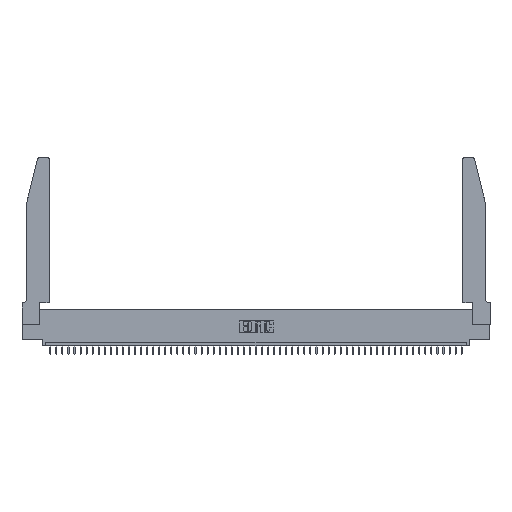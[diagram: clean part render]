
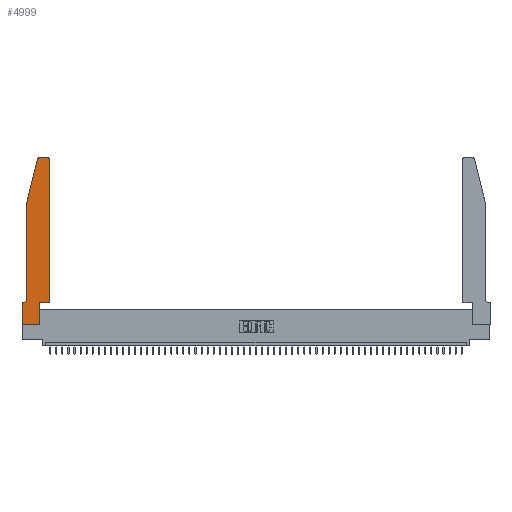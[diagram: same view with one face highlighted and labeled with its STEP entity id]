
A CAD part, top view. The second image highlights one B-rep face of the part: STEP entity #4999.
In plain terms, the highlighted planar face has unit normal (0, 0, 1).
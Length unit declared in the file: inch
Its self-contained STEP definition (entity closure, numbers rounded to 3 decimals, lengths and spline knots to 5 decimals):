
#394 = CARTESIAN_POINT ( 'NONE',  ( 0.0755, 2., 0.37 ) ) ;
#977 = EDGE_CURVE ( 'NONE', #12827, #989, #22823, .T. ) ;
#989 = VERTEX_POINT ( 'NONE', #33174 ) ;
#1142 = AXIS2_PLACEMENT_3D ( 'NONE', #29345, #42253, #9638 ) ;
#1189 = EDGE_CURVE ( 'NONE', #13287, #12827, #1862, .T. ) ;
#1862 = LINE ( 'NONE', #22074, #22867 ) ;
#1951 = DIRECTION ( 'NONE',  ( -1., 0., 0. ) ) ;
#2923 = DIRECTION ( 'NONE',  ( 1., 0., 0. ) ) ;
#4342 = DIRECTION ( 'NONE',  ( 1., 0., 0. ) ) ;
#4626 = VERTEX_POINT ( 'NONE', #16814 ) ;
#4999 = ADVANCED_FACE ( 'NONE', ( #16238 ), #24892, .T. ) ;
#5013 = LINE ( 'NONE', #41927, #43911 ) ;
#5297 = DIRECTION ( 'NONE',  ( -0.239, -0.971, 0. ) ) ;
#5701 = VERTEX_POINT ( 'NONE', #25936 ) ;
#7807 = EDGE_CURVE ( 'NONE', #13977, #37453, #43883, .T. ) ;
#7870 = CARTESIAN_POINT ( 'NONE',  ( 0.4505, 0.35, 0.37 ) ) ;
#8612 = ORIENTED_EDGE ( 'NONE', *, *, #1189, .T. ) ;
#8621 = VERTEX_POINT ( 'NONE', #28650 ) ;
#8873 = EDGE_CURVE ( 'NONE', #20160, #5701, #52295, .T. ) ;
#8943 = ORIENTED_EDGE ( 'NONE', *, *, #35879, .T. ) ;
#9638 = DIRECTION ( 'NONE',  ( 1., 0., 0. ) ) ;
#10596 = EDGE_CURVE ( 'NONE', #41810, #4626, #53225, .T. ) ;
#10607 = CIRCLE ( 'NONE', #1142, 0.03 ) ;
#10634 = VECTOR ( 'NONE', #29252, 39.37008 ) ;
#11757 = CARTESIAN_POINT ( 'NONE',  ( 0., 0., 0.37 ) ) ;
#12827 = VERTEX_POINT ( 'NONE', #26714 ) ;
#13287 = VERTEX_POINT ( 'NONE', #30413 ) ;
#13802 = CARTESIAN_POINT ( 'NONE',  ( 0.4505, 0.35, 0.37 ) ) ;
#13977 = VERTEX_POINT ( 'NONE', #50660 ) ;
#14896 = EDGE_CURVE ( 'NONE', #30742, #8621, #15386, .T. ) ;
#15386 = LINE ( 'NONE', #7870, #46083 ) ;
#16238 = FACE_OUTER_BOUND ( 'NONE', #37562, .T. ) ;
#16446 = CARTESIAN_POINT ( 'NONE',  ( 0., 0., 0.37 ) ) ;
#16768 = AXIS2_PLACEMENT_3D ( 'NONE', #46085, #28875, #4342 ) ;
#16814 = CARTESIAN_POINT ( 'NONE',  ( 0., 0.35, 0.37 ) ) ;
#17313 = LINE ( 'NONE', #13802, #19300 ) ;
#18784 = CARTESIAN_POINT ( 'NONE',  ( 0.0055, 0.35, 0.37 ) ) ;
#19300 = VECTOR ( 'NONE', #49950, 39.37008 ) ;
#20160 = VERTEX_POINT ( 'NONE', #394 ) ;
#20264 = DIRECTION ( 'NONE',  ( 0., 1., 0. ) ) ;
#20481 = VECTOR ( 'NONE', #2923, 39.37008 ) ;
#20873 = ORIENTED_EDGE ( 'NONE', *, *, #977, .T. ) ;
#21095 = DIRECTION ( 'NONE',  ( 1., 0., 0. ) ) ;
#21529 = LINE ( 'NONE', #26131, #34933 ) ;
#22074 = CARTESIAN_POINT ( 'NONE',  ( 0.2605, 2.75, 0.37 ) ) ;
#22645 = EDGE_CURVE ( 'NONE', #5701, #41810, #32778, .T. ) ;
#22823 = CIRCLE ( 'NONE', #16768, 0.03 ) ;
#22867 = VECTOR ( 'NONE', #22886, 39.37008 ) ;
#22886 = DIRECTION ( 'NONE',  ( -1., 0., 0. ) ) ;
#24339 = VECTOR ( 'NONE', #44229, 39.37008 ) ;
#24705 = VECTOR ( 'NONE', #36691, 39.37008 ) ;
#24892 = PLANE ( 'NONE',  #42009 ) ;
#25166 = CARTESIAN_POINT ( 'NONE',  ( 0., 0.35, 0.37 ) ) ;
#25936 = CARTESIAN_POINT ( 'NONE',  ( 0.0755, 0.42, 0.37 ) ) ;
#26131 = CARTESIAN_POINT ( 'NONE',  ( 0.2865, 0.35, 0.37 ) ) ;
#26133 = ORIENTED_EDGE ( 'NONE', *, *, #8873, .T. ) ;
#26192 = CARTESIAN_POINT ( 'NONE',  ( 0.4505, 0.35, 0.37 ) ) ;
#26714 = CARTESIAN_POINT ( 'NONE',  ( 0.284, 2.75, 0.37 ) ) ;
#27071 = EDGE_CURVE ( 'NONE', #989, #20160, #5013, .T. ) ;
#28650 = CARTESIAN_POINT ( 'NONE',  ( 0.4505, 2.72, 0.37 ) ) ;
#28875 = DIRECTION ( 'NONE',  ( 0., 0., 1. ) ) ;
#29252 = DIRECTION ( 'NONE',  ( -1., 0., 0. ) ) ;
#29345 = CARTESIAN_POINT ( 'NONE',  ( 0.4205, 2.72, 0.37 ) ) ;
#29885 = DIRECTION ( 'NONE',  ( 0., 1., 0. ) ) ;
#30049 = ORIENTED_EDGE ( 'NONE', *, *, #33346, .T. ) ;
#30413 = CARTESIAN_POINT ( 'NONE',  ( 0.4205, 2.75, 0.37 ) ) ;
#30742 = VERTEX_POINT ( 'NONE', #26192 ) ;
#31067 = CARTESIAN_POINT ( 'NONE',  ( 0.0055, 0.42, 0.37 ) ) ;
#32384 = CARTESIAN_POINT ( 'NONE',  ( 0.2865, 0., 0.37 ) ) ;
#32778 = CIRCLE ( 'NONE', #37937, 0.07 ) ;
#32915 = LINE ( 'NONE', #16446, #24705 ) ;
#33011 = ORIENTED_EDGE ( 'NONE', *, *, #38864, .T. ) ;
#33017 = CARTESIAN_POINT ( 'NONE',  ( 0.0755, 0.35, 0.37 ) ) ;
#33025 = ORIENTED_EDGE ( 'NONE', *, *, #14896, .T. ) ;
#33174 = CARTESIAN_POINT ( 'NONE',  ( 0.25487, 2.72718, 0.37 ) ) ;
#33346 = EDGE_CURVE ( 'NONE', #8621, #13287, #10607, .T. ) ;
#34833 = DIRECTION ( 'NONE',  ( 0., 0., -1. ) ) ;
#34933 = VECTOR ( 'NONE', #29885, 39.37008 ) ;
#35879 = EDGE_CURVE ( 'NONE', #37453, #48355, #21529, .T. ) ;
#36307 = ORIENTED_EDGE ( 'NONE', *, *, #27071, .T. ) ;
#36691 = DIRECTION ( 'NONE',  ( 0., -1., 0. ) ) ;
#37453 = VERTEX_POINT ( 'NONE', #32384 ) ;
#37562 = EDGE_LOOP ( 'NONE', ( #8612, #20873, #36307, #26133, #39163, #40458, #33011, #46998, #8943, #52163, #33025, #30049 ) ) ;
#37937 = AXIS2_PLACEMENT_3D ( 'NONE', #31067, #34833, #1951 ) ;
#38864 = EDGE_CURVE ( 'NONE', #4626, #13977, #32915, .T. ) ;
#39163 = ORIENTED_EDGE ( 'NONE', *, *, #22645, .T. ) ;
#40458 = ORIENTED_EDGE ( 'NONE', *, *, #10596, .T. ) ;
#41810 = VERTEX_POINT ( 'NONE', #18784 ) ;
#41927 = CARTESIAN_POINT ( 'NONE',  ( 0.0755, 2., 0.37 ) ) ;
#42009 = AXIS2_PLACEMENT_3D ( 'NONE', #25166, #45106, #21095 ) ;
#42253 = DIRECTION ( 'NONE',  ( 0., 0., 1. ) ) ;
#43883 = LINE ( 'NONE', #11757, #20481 ) ;
#43911 = VECTOR ( 'NONE', #5297, 39.37008 ) ;
#44229 = DIRECTION ( 'NONE',  ( 0., -1., 0. ) ) ;
#45106 = DIRECTION ( 'NONE',  ( 0., 0., 1. ) ) ;
#45418 = CARTESIAN_POINT ( 'NONE',  ( 0.2865, 0.35, 0.37 ) ) ;
#46083 = VECTOR ( 'NONE', #20264, 39.37008 ) ;
#46085 = CARTESIAN_POINT ( 'NONE',  ( 0.284, 2.72, 0.37 ) ) ;
#46998 = ORIENTED_EDGE ( 'NONE', *, *, #7807, .T. ) ;
#47993 = CARTESIAN_POINT ( 'NONE',  ( 0.0755, 2., 0.37 ) ) ;
#48355 = VERTEX_POINT ( 'NONE', #45418 ) ;
#48929 = EDGE_CURVE ( 'NONE', #48355, #30742, #17313, .T. ) ;
#49950 = DIRECTION ( 'NONE',  ( 1., 0., 0. ) ) ;
#50660 = CARTESIAN_POINT ( 'NONE',  ( 0., 0., 0.37 ) ) ;
#52163 = ORIENTED_EDGE ( 'NONE', *, *, #48929, .T. ) ;
#52295 = LINE ( 'NONE', #47993, #24339 ) ;
#53225 = LINE ( 'NONE', #33017, #10634 ) ;
